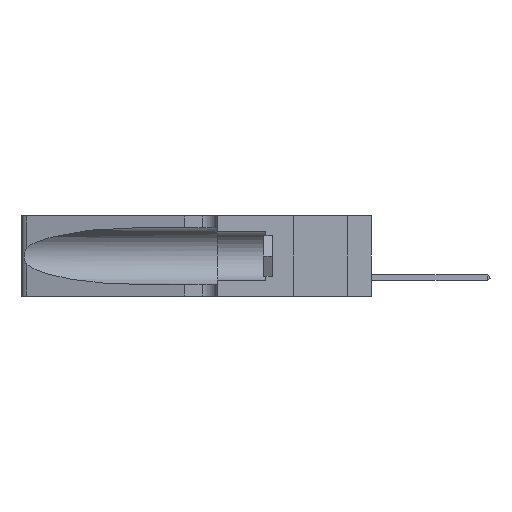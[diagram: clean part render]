
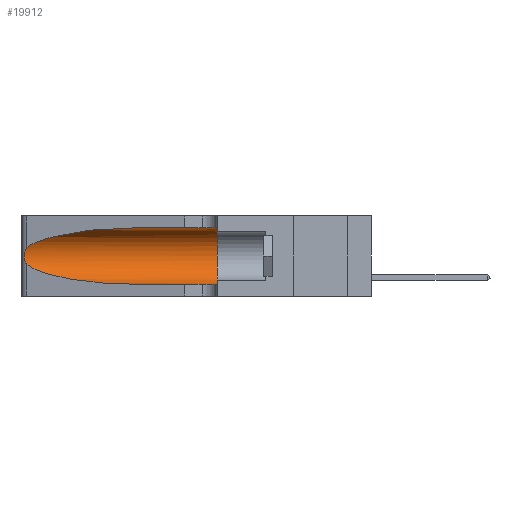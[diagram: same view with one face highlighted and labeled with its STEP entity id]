
A CAD part, left-side view. The second image highlights one B-rep face of the part: STEP entity #19912.
In plain terms, the highlighted cylindrical face has radius 3.308 mm (diameter 6.617 mm), a partial arc.
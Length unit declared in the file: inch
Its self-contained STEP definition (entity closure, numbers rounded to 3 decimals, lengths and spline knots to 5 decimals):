
#433 = CARTESIAN_POINT ( 'NONE',  ( 0.25639, 1.23186, 0.15144 ) ) ;
#619 = EDGE_CURVE ( 'NONE', #10647, #6796, #3552, .T. ) ;
#1371 = CARTESIAN_POINT ( 'NONE',  ( 0.1305, 1.61858, 0.05475 ) ) ;
#1409 = LINE ( 'NONE', #22191, #18557 ) ;
#1437 = DIRECTION ( 'NONE',  ( 0., 0., 1. ) ) ;
#1880 = EDGE_CURVE ( 'NONE', #16762, #17385, #14497, .T. ) ;
#2145 = CARTESIAN_POINT ( 'NONE',  ( 0.25854, 1.2359, 0.20912 ) ) ;
#2194 = CARTESIAN_POINT ( 'NONE',  ( 0.1305, 0.72297, 0.05475 ) ) ;
#2310 = EDGE_CURVE ( 'NONE', #6796, #6697, #7148, .T. ) ;
#2821 = CYLINDRICAL_SURFACE ( 'NONE', #11304, 0.13025 ) ;
#3075 = ORIENTED_EDGE ( 'NONE', *, *, #1880, .F. ) ;
#3552 =( BOUNDED_CURVE ( )  B_SPLINE_CURVE ( 3, ( #20958, #17639, #19498, #12392 ),
 .UNSPECIFIED., .F., .F. ) 
 B_SPLINE_CURVE_WITH_KNOTS ( ( 4, 4 ),
 ( 1.5708, 2.84003 ),
 .UNSPECIFIED. ) 
 CURVE ( )  GEOMETRIC_REPRESENTATION_ITEM ( )  RATIONAL_B_SPLINE_CURVE ( ( 1., 0.87, 0.87, 1. ) ) 
 REPRESENTATION_ITEM ( '' )  );
#3725 = CARTESIAN_POINT ( 'NONE',  ( 0.25789, 1.23486, 0.15765 ) ) ;
#4113 = ORIENTED_EDGE ( 'NONE', *, *, #10220, .T. ) ;
#4809 = CARTESIAN_POINT ( 'NONE',  ( 0.2373, 1.15595, 0.08982 ) ) ;
#5374 = CARTESIAN_POINT ( 'NONE',  ( 0.25555, 1.22994, 0.2215 ) ) ;
#5450 = CARTESIAN_POINT ( 'NONE',  ( 0.25555, 1.22993, 0.14849 ) ) ;
#6222 = CARTESIAN_POINT ( 'NONE',  ( 0.1305, 1.61858, 0.185 ) ) ;
#6459 = CARTESIAN_POINT ( 'NONE',  ( 0.25487, 1.22718, 0.14631 ) ) ;
#6697 = VERTEX_POINT ( 'NONE', #17386 ) ;
#6746 = ORIENTED_EDGE ( 'NONE', *, *, #15245, .F. ) ;
#6796 = VERTEX_POINT ( 'NONE', #16193 ) ;
#7148 = B_SPLINE_CURVE_WITH_KNOTS ( 'NONE', 3,
 ( #13992, #5374, #7405, #8970, #2145, #17312, #10654, #7258, #15651, #10578, #3725, #433, #5450, #15724 ),
 .UNSPECIFIED., .F., .F.,
 ( 4, 2, 2, 2, 2, 2, 4 ),
 ( 0., 0.00027, 0.00053, 0.00107, 0.0016, 0.00187, 0.00214 ),
 .UNSPECIFIED. ) ;
#7258 = CARTESIAN_POINT ( 'NONE',  ( 0.26075, 1.23896, 0.178 ) ) ;
#7405 = CARTESIAN_POINT ( 'NONE',  ( 0.25639, 1.23184, 0.21858 ) ) ;
#7781 = ORIENTED_EDGE ( 'NONE', *, *, #12827, .T. ) ;
#8256 = DIRECTION ( 'NONE',  ( 0., -1., 0. ) ) ;
#8970 = CARTESIAN_POINT ( 'NONE',  ( 0.25787, 1.23484, 0.2124 ) ) ;
#9494 = VERTEX_POINT ( 'NONE', #2194 ) ;
#9662 = DIRECTION ( 'NONE',  ( 0., -1., 0. ) ) ;
#10118 =( BOUNDED_CURVE ( )  B_SPLINE_CURVE ( 3, ( #6459, #4809, #18480, #21813 ),
 .UNSPECIFIED., .F., .T. ) 
 B_SPLINE_CURVE_WITH_KNOTS ( ( 4, 4 ),
 ( 3.44316, 4.71239 ),
 .UNSPECIFIED. ) 
 CURVE ( )  GEOMETRIC_REPRESENTATION_ITEM ( )  RATIONAL_B_SPLINE_CURVE ( ( 1., 0.87, 0.87, 1. ) ) 
 REPRESENTATION_ITEM ( '' )  );
#10220 = EDGE_CURVE ( 'NONE', #9494, #17385, #15441, .T. ) ;
#10578 = CARTESIAN_POINT ( 'NONE',  ( 0.25856, 1.23593, 0.16098 ) ) ;
#10647 = VERTEX_POINT ( 'NONE', #21065 ) ;
#10654 = CARTESIAN_POINT ( 'NONE',  ( 0.26075, 1.23896, 0.19203 ) ) ;
#11304 = AXIS2_PLACEMENT_3D ( 'NONE', #6222, #9662, #19830 ) ;
#12392 = CARTESIAN_POINT ( 'NONE',  ( 0.25487, 1.22718, 0.22369 ) ) ;
#12827 = EDGE_CURVE ( 'NONE', #6697, #9494, #10118, .T. ) ;
#13008 = CARTESIAN_POINT ( 'NONE',  ( 0.1305, 0.35, 0.05475 ) ) ;
#13288 = CARTESIAN_POINT ( 'NONE',  ( 0.1305, 0.35, 0.185 ) ) ;
#13386 = ORIENTED_EDGE ( 'NONE', *, *, #2310, .T. ) ;
#13992 = CARTESIAN_POINT ( 'NONE',  ( 0.25487, 1.22718, 0.22369 ) ) ;
#14060 = AXIS2_PLACEMENT_3D ( 'NONE', #13288, #20209, #1437 ) ;
#14151 = ORIENTED_EDGE ( 'NONE', *, *, #619, .T. ) ;
#14497 = CIRCLE ( 'NONE', #14060, 0.13025 ) ;
#15245 = EDGE_CURVE ( 'NONE', #10647, #16762, #1409, .T. ) ;
#15441 = LINE ( 'NONE', #1371, #17076 ) ;
#15651 = CARTESIAN_POINT ( 'NONE',  ( 0.26017, 1.23833, 0.17102 ) ) ;
#15724 = CARTESIAN_POINT ( 'NONE',  ( 0.25487, 1.22718, 0.14631 ) ) ;
#16193 = CARTESIAN_POINT ( 'NONE',  ( 0.25487, 1.22718, 0.22369 ) ) ;
#16213 = EDGE_LOOP ( 'NONE', ( #14151, #13386, #7781, #4113, #3075, #6746 ) ) ;
#16762 = VERTEX_POINT ( 'NONE', #18962 ) ;
#17076 = VECTOR ( 'NONE', #18498, 39.37008 ) ;
#17312 = CARTESIAN_POINT ( 'NONE',  ( 0.26018, 1.23835, 0.19895 ) ) ;
#17385 = VERTEX_POINT ( 'NONE', #13008 ) ;
#17386 = CARTESIAN_POINT ( 'NONE',  ( 0.25487, 1.22718, 0.14631 ) ) ;
#17639 = CARTESIAN_POINT ( 'NONE',  ( 0.18966, 0.96281, 0.31525 ) ) ;
#18480 = CARTESIAN_POINT ( 'NONE',  ( 0.18966, 0.96281, 0.05475 ) ) ;
#18498 = DIRECTION ( 'NONE',  ( 0., -1., 0. ) ) ;
#18557 = VECTOR ( 'NONE', #8256, 39.37008 ) ;
#18608 = FACE_OUTER_BOUND ( 'NONE', #16213, .T. ) ;
#18962 = CARTESIAN_POINT ( 'NONE',  ( 0.1305, 0.35, 0.31525 ) ) ;
#19498 = CARTESIAN_POINT ( 'NONE',  ( 0.2373, 1.15595, 0.28018 ) ) ;
#19830 = DIRECTION ( 'NONE',  ( 0., 0., -1. ) ) ;
#19912 = ADVANCED_FACE ( 'NONE', ( #18608 ), #2821, .F. ) ;
#20209 = DIRECTION ( 'NONE',  ( 0., 1., 0. ) ) ;
#20958 = CARTESIAN_POINT ( 'NONE',  ( 0.1305, 0.72297, 0.31525 ) ) ;
#21065 = CARTESIAN_POINT ( 'NONE',  ( 0.1305, 0.72297, 0.31525 ) ) ;
#21813 = CARTESIAN_POINT ( 'NONE',  ( 0.1305, 0.72297, 0.05475 ) ) ;
#22191 = CARTESIAN_POINT ( 'NONE',  ( 0.1305, 1.61858, 0.31525 ) ) ;
